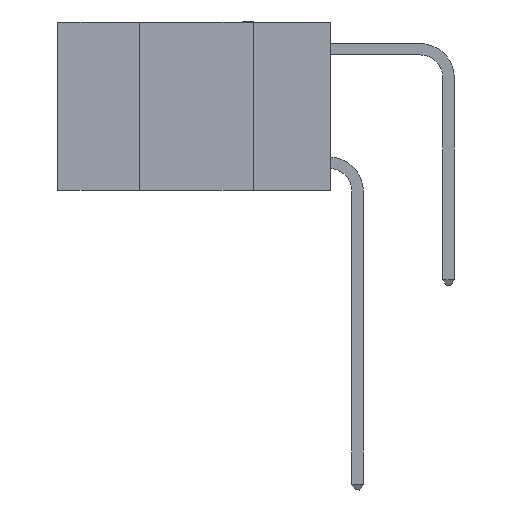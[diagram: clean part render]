
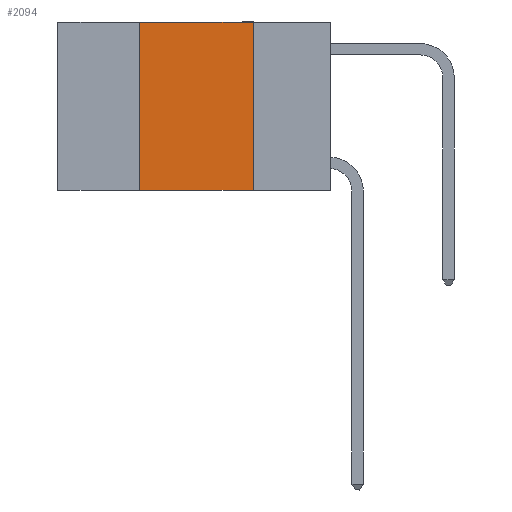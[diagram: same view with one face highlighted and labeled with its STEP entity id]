
A CAD part, left-side view. The second image highlights one B-rep face of the part: STEP entity #2094.
In plain terms, the highlighted planar face has unit normal (-1, 0, 0).
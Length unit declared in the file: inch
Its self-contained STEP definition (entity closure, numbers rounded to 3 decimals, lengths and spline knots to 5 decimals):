
#2012 = CARTESIAN_POINT ( 'NONE',  ( 0., 0.17, 0. ) ) ;
#2094 = ADVANCED_FACE ( 'NONE', ( #13115 ), #23413, .F. ) ;
#3036 = DIRECTION ( 'NONE',  ( 0., -1., 0. ) ) ;
#3158 = CARTESIAN_POINT ( 'NONE',  ( 0., 0.17, 0. ) ) ;
#4082 = CARTESIAN_POINT ( 'NONE',  ( 0., 0.42, -0.37 ) ) ;
#4085 = LINE ( 'NONE', #16563, #18761 ) ;
#4088 = ORIENTED_EDGE ( 'NONE', *, *, #15185, .F. ) ;
#4568 = DIRECTION ( 'NONE',  ( 0., 0., -1. ) ) ;
#4765 = CARTESIAN_POINT ( 'NONE',  ( 0., 0.42, 0. ) ) ;
#5375 = ORIENTED_EDGE ( 'NONE', *, *, #11304, .F. ) ;
#5905 = VERTEX_POINT ( 'NONE', #4082 ) ;
#5988 = CARTESIAN_POINT ( 'NONE',  ( 0., 0.42, 0. ) ) ;
#7699 = ORIENTED_EDGE ( 'NONE', *, *, #15440, .F. ) ;
#8197 = AXIS2_PLACEMENT_3D ( 'NONE', #19739, #16126, #4568 ) ;
#8486 = VERTEX_POINT ( 'NONE', #18979 ) ;
#8708 = DIRECTION ( 'NONE',  ( 0., -1., 0. ) ) ;
#10502 = VECTOR ( 'NONE', #20344, 39.37008 ) ;
#10732 = ORIENTED_EDGE ( 'NONE', *, *, #15443, .T. ) ;
#10799 = VECTOR ( 'NONE', #18176, 39.37008 ) ;
#11112 = LINE ( 'NONE', #3158, #10502 ) ;
#11304 = EDGE_CURVE ( 'NONE', #17037, #17033, #4085, .T. ) ;
#13115 = FACE_OUTER_BOUND ( 'NONE', #21491, .T. ) ;
#14381 = CARTESIAN_POINT ( 'NONE',  ( 0., 0.6, -0.37 ) ) ;
#15185 = EDGE_CURVE ( 'NONE', #17033, #8486, #11112, .T. ) ;
#15250 = LINE ( 'NONE', #4765, #10799 ) ;
#15440 = EDGE_CURVE ( 'NONE', #5905, #17037, #15250, .T. ) ;
#15443 = EDGE_CURVE ( 'NONE', #5905, #8486, #16483, .T. ) ;
#16126 = DIRECTION ( 'NONE',  ( 1., 0., 0. ) ) ;
#16483 = LINE ( 'NONE', #14381, #19604 ) ;
#16563 = CARTESIAN_POINT ( 'NONE',  ( 0., 0.6, 0. ) ) ;
#17033 = VERTEX_POINT ( 'NONE', #2012 ) ;
#17037 = VERTEX_POINT ( 'NONE', #5988 ) ;
#18176 = DIRECTION ( 'NONE',  ( 0., 0., 1. ) ) ;
#18761 = VECTOR ( 'NONE', #3036, 39.37008 ) ;
#18979 = CARTESIAN_POINT ( 'NONE',  ( 0., 0.17, -0.37 ) ) ;
#19604 = VECTOR ( 'NONE', #8708, 39.37008 ) ;
#19739 = CARTESIAN_POINT ( 'NONE',  ( 0., 0.6, 0. ) ) ;
#20344 = DIRECTION ( 'NONE',  ( 0., 0., -1. ) ) ;
#21491 = EDGE_LOOP ( 'NONE', ( #4088, #5375, #7699, #10732 ) ) ;
#23413 = PLANE ( 'NONE',  #8197 ) ;
